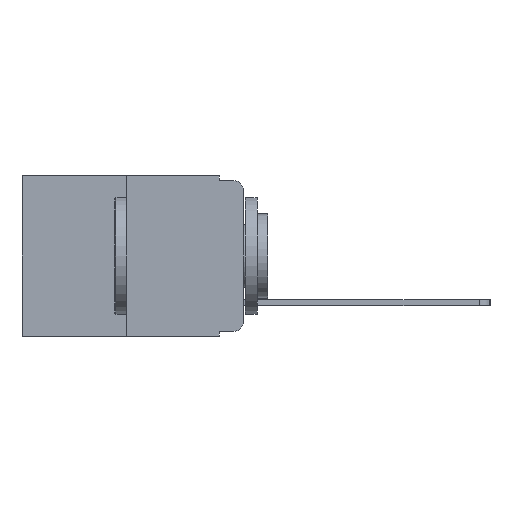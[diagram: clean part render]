
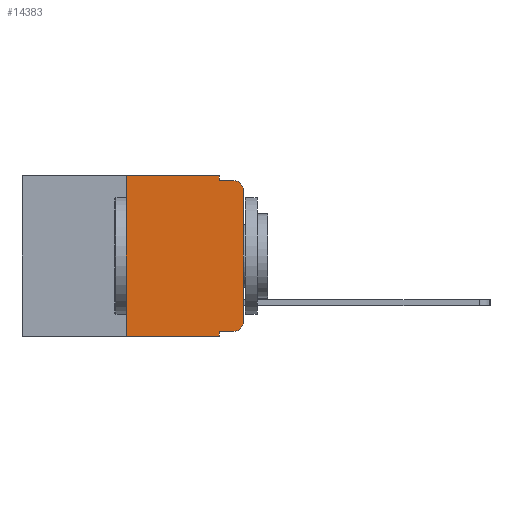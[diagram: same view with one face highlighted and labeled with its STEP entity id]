
A CAD part, left-side view. The second image highlights one B-rep face of the part: STEP entity #14383.
In plain terms, the highlighted planar face has unit normal (-1, 0, 0).
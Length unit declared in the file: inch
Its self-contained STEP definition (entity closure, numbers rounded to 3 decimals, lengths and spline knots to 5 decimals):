
#205 = EDGE_CURVE ( 'NONE', #7232, #4035, #17079, .T. ) ;
#489 = EDGE_CURVE ( 'NONE', #7125, #2593, #15984, .T. ) ;
#736 = ORIENTED_EDGE ( 'NONE', *, *, #16992, .F. ) ;
#770 = ORIENTED_EDGE ( 'NONE', *, *, #489, .T. ) ;
#794 = ORIENTED_EDGE ( 'NONE', *, *, #15134, .F. ) ;
#814 = CARTESIAN_POINT ( 'NONE',  ( 0., 0.25, 0. ) ) ;
#1102 = CARTESIAN_POINT ( 'NONE',  ( 0., 0.051, -0.343 ) ) ;
#1124 = AXIS2_PLACEMENT_3D ( 'NONE', #2922, #12983, #4438 ) ;
#1187 = ORIENTED_EDGE ( 'NONE', *, *, #13388, .F. ) ;
#1210 = AXIS2_PLACEMENT_3D ( 'NONE', #3017, #13074, #4528 ) ;
#1972 = CARTESIAN_POINT ( 'NONE',  ( 0., 0., 0. ) ) ;
#2243 = EDGE_CURVE ( 'NONE', #17773, #4035, #17631, .T. ) ;
#2482 = VERTEX_POINT ( 'NONE', #2819 ) ;
#2493 = ORIENTED_EDGE ( 'NONE', *, *, #13245, .T. ) ;
#2593 = VERTEX_POINT ( 'NONE', #1102 ) ;
#2611 = EDGE_LOOP ( 'NONE', ( #18413, #15796, #16790, #18543, #1187, #736, #770, #794, #2493, #2969 ) ) ;
#2819 = CARTESIAN_POINT ( 'NONE',  ( 0., 0.051, 0. ) ) ;
#2922 = CARTESIAN_POINT ( 'NONE',  ( 0., 0.473, 0. ) ) ;
#2962 = CARTESIAN_POINT ( 'NONE',  ( 0., 0.051, 0. ) ) ;
#2969 = ORIENTED_EDGE ( 'NONE', *, *, #11361, .T. ) ;
#3017 = CARTESIAN_POINT ( 'NONE',  ( 0., 0.02, -0.313 ) ) ;
#3088 = DIRECTION ( 'NONE',  ( 0., 0., 1. ) ) ;
#3256 = EDGE_CURVE ( 'NONE', #7389, #17773, #15736, .T. ) ;
#3260 = CARTESIAN_POINT ( 'NONE',  ( 0., 0.473, 0. ) ) ;
#4035 = VERTEX_POINT ( 'NONE', #16921 ) ;
#4369 = PLANE ( 'NONE',  #1124 ) ;
#4438 = DIRECTION ( 'NONE',  ( 0., 0., -1. ) ) ;
#4523 = CARTESIAN_POINT ( 'NONE',  ( 0., 0.051, -0.01 ) ) ;
#4528 = DIRECTION ( 'NONE',  ( 0., 0., -1. ) ) ;
#5047 = CARTESIAN_POINT ( 'NONE',  ( 0., 0., -0.03 ) ) ;
#5200 = LINE ( 'NONE', #5895, #12305 ) ;
#5306 = DIRECTION ( 'NONE',  ( 0., 0., -1. ) ) ;
#5760 = VERTEX_POINT ( 'NONE', #12642 ) ;
#5895 = CARTESIAN_POINT ( 'NONE',  ( 0., 0.051, -0.333 ) ) ;
#5955 = DIRECTION ( 'NONE',  ( 0., -1., 0. ) ) ;
#6006 = VERTEX_POINT ( 'NONE', #9000 ) ;
#6091 = CARTESIAN_POINT ( 'NONE',  ( 0., 0.25, 0. ) ) ;
#6315 = DIRECTION ( 'NONE',  ( -1., 0., 0. ) ) ;
#6340 = CARTESIAN_POINT ( 'NONE',  ( 0., 0.02, -0.03 ) ) ;
#6341 = VECTOR ( 'NONE', #13320, 39.37008 ) ;
#6708 = LINE ( 'NONE', #6775, #17432 ) ;
#6775 = CARTESIAN_POINT ( 'NONE',  ( 0., 0.051, 0. ) ) ;
#7125 = VERTEX_POINT ( 'NONE', #15643 ) ;
#7232 = VERTEX_POINT ( 'NONE', #4523 ) ;
#7389 = VERTEX_POINT ( 'NONE', #10549 ) ;
#7663 = VECTOR ( 'NONE', #8835, 39.37008 ) ;
#8315 = LINE ( 'NONE', #2962, #7663 ) ;
#8835 = DIRECTION ( 'NONE',  ( 0., 0., -1. ) ) ;
#9000 = CARTESIAN_POINT ( 'NONE',  ( 0., 0.051, -0.333 ) ) ;
#9555 = LINE ( 'NONE', #6091, #16551 ) ;
#10108 = LINE ( 'NONE', #3260, #6341 ) ;
#10549 = CARTESIAN_POINT ( 'NONE',  ( 0., 0., -0.313 ) ) ;
#11361 = EDGE_CURVE ( 'NONE', #5760, #7389, #14901, .T. ) ;
#12222 = DIRECTION ( 'NONE',  ( 0., -1., 0. ) ) ;
#12256 = VECTOR ( 'NONE', #15824, 39.37008 ) ;
#12305 = VECTOR ( 'NONE', #5955, 39.37008 ) ;
#12642 = CARTESIAN_POINT ( 'NONE',  ( 0., 0.02, -0.333 ) ) ;
#12821 = CARTESIAN_POINT ( 'NONE',  ( 0., 0.051, -0.01 ) ) ;
#12983 = DIRECTION ( 'NONE',  ( 1., 0., 0. ) ) ;
#13074 = DIRECTION ( 'NONE',  ( -1., 0., 0. ) ) ;
#13109 = CARTESIAN_POINT ( 'NONE',  ( 0., 0.473, -0.343 ) ) ;
#13245 = EDGE_CURVE ( 'NONE', #6006, #5760, #5200, .T. ) ;
#13320 = DIRECTION ( 'NONE',  ( 0., -1., 0. ) ) ;
#13388 = EDGE_CURVE ( 'NONE', #17905, #2482, #10108, .T. ) ;
#13810 = VECTOR ( 'NONE', #12222, 39.37008 ) ;
#14383 = ADVANCED_FACE ( 'NONE', ( #18511 ), #4369, .F. ) ;
#14901 = CIRCLE ( 'NONE', #1210, 0.02 ) ;
#15134 = EDGE_CURVE ( 'NONE', #6006, #2593, #8315, .T. ) ;
#15189 = DIRECTION ( 'NONE',  ( 0., 0., -1. ) ) ;
#15299 = VECTOR ( 'NONE', #18324, 39.37008 ) ;
#15643 = CARTESIAN_POINT ( 'NONE',  ( 0., 0.25, -0.343 ) ) ;
#15736 = LINE ( 'NONE', #1972, #15299 ) ;
#15796 = ORIENTED_EDGE ( 'NONE', *, *, #2243, .T. ) ;
#15824 = DIRECTION ( 'NONE',  ( 0., -1., 0. ) ) ;
#15984 = LINE ( 'NONE', #13109, #12256 ) ;
#16185 = AXIS2_PLACEMENT_3D ( 'NONE', #6340, #6315, #15189 ) ;
#16551 = VECTOR ( 'NONE', #3088, 39.37008 ) ;
#16790 = ORIENTED_EDGE ( 'NONE', *, *, #205, .F. ) ;
#16921 = CARTESIAN_POINT ( 'NONE',  ( 0., 0.02, -0.01 ) ) ;
#16992 = EDGE_CURVE ( 'NONE', #7125, #17905, #9555, .T. ) ;
#17079 = LINE ( 'NONE', #12821, #13810 ) ;
#17432 = VECTOR ( 'NONE', #5306, 39.37008 ) ;
#17631 = CIRCLE ( 'NONE', #16185, 0.02 ) ;
#17773 = VERTEX_POINT ( 'NONE', #5047 ) ;
#17898 = EDGE_CURVE ( 'NONE', #2482, #7232, #6708, .T. ) ;
#17905 = VERTEX_POINT ( 'NONE', #814 ) ;
#18324 = DIRECTION ( 'NONE',  ( 0., 0., 1. ) ) ;
#18413 = ORIENTED_EDGE ( 'NONE', *, *, #3256, .T. ) ;
#18511 = FACE_OUTER_BOUND ( 'NONE', #2611, .T. ) ;
#18543 = ORIENTED_EDGE ( 'NONE', *, *, #17898, .F. ) ;
